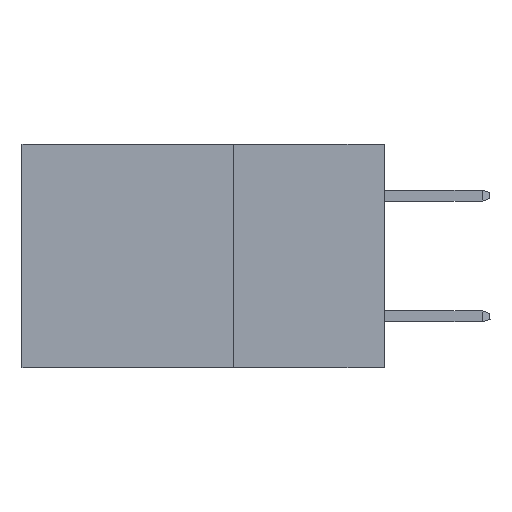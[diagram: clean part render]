
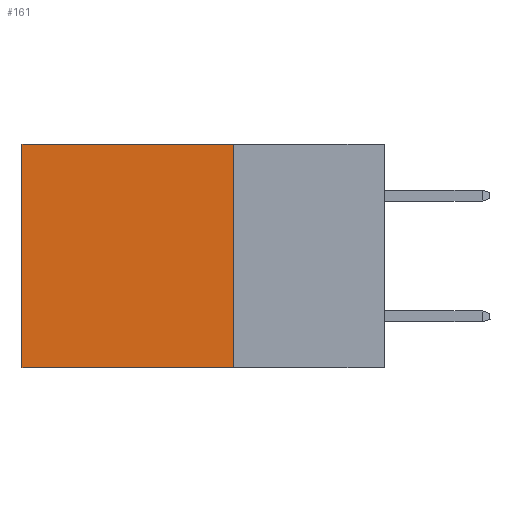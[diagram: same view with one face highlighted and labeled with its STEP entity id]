
A CAD part, left-side view. The second image highlights one B-rep face of the part: STEP entity #161.
In plain terms, the highlighted planar face has unit normal (-1, 0, 0).
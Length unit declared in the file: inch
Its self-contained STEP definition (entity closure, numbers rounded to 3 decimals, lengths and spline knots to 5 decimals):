
#161 = ADVANCED_FACE ( 'NONE', ( #3444 ), #9119, .F. ) ;
#740 = VERTEX_POINT ( 'NONE', #3530 ) ;
#1201 = VERTEX_POINT ( 'NONE', #7461 ) ;
#1665 = AXIS2_PLACEMENT_3D ( 'NONE', #10880, #9931, #5651 ) ;
#2228 = CARTESIAN_POINT ( 'NONE',  ( 0.2615, 0.6, -0.37 ) ) ;
#2464 = CARTESIAN_POINT ( 'NONE',  ( 0.2615, 0.25, -0.37 ) ) ;
#3444 = FACE_OUTER_BOUND ( 'NONE', #10472, .T. ) ;
#3530 = CARTESIAN_POINT ( 'NONE',  ( 0.2615, 0.6, 0. ) ) ;
#3645 = LINE ( 'NONE', #2464, #8260 ) ;
#3822 = VECTOR ( 'NONE', #5399, 39.37008 ) ;
#4147 = ORIENTED_EDGE ( 'NONE', *, *, #4760, .T. ) ;
#4585 = CARTESIAN_POINT ( 'NONE',  ( 0.2615, 0.25, 0. ) ) ;
#4722 = VERTEX_POINT ( 'NONE', #4585 ) ;
#4760 = EDGE_CURVE ( 'NONE', #4722, #740, #6684, .T. ) ;
#5399 = DIRECTION ( 'NONE',  ( 0., 1., 0. ) ) ;
#5562 = EDGE_CURVE ( 'NONE', #8743, #1201, #8564, .T. ) ;
#5651 = DIRECTION ( 'NONE',  ( 0., 0., -1. ) ) ;
#6229 = ORIENTED_EDGE ( 'NONE', *, *, #6980, .T. ) ;
#6668 = CARTESIAN_POINT ( 'NONE',  ( 0.2615, 0.25, -0.37 ) ) ;
#6683 = DIRECTION ( 'NONE',  ( 0., 0., -1. ) ) ;
#6684 = LINE ( 'NONE', #7137, #3822 ) ;
#6980 = EDGE_CURVE ( 'NONE', #740, #1201, #11084, .T. ) ;
#7137 = CARTESIAN_POINT ( 'NONE',  ( 0.2615, 0.25, 0. ) ) ;
#7321 = CARTESIAN_POINT ( 'NONE',  ( 0.2615, 0.25, -0.37 ) ) ;
#7461 = CARTESIAN_POINT ( 'NONE',  ( 0.2615, 0.6, -0.37 ) ) ;
#8260 = VECTOR ( 'NONE', #8625, 39.37008 ) ;
#8398 = DIRECTION ( 'NONE',  ( 0., 1., 0. ) ) ;
#8564 = LINE ( 'NONE', #6668, #10363 ) ;
#8625 = DIRECTION ( 'NONE',  ( 0., 0., -1. ) ) ;
#8743 = VERTEX_POINT ( 'NONE', #7321 ) ;
#8790 = ORIENTED_EDGE ( 'NONE', *, *, #10725, .F. ) ;
#9119 = PLANE ( 'NONE',  #1665 ) ;
#9484 = ORIENTED_EDGE ( 'NONE', *, *, #5562, .F. ) ;
#9931 = DIRECTION ( 'NONE',  ( 1., 0., 0. ) ) ;
#10363 = VECTOR ( 'NONE', #8398, 39.37008 ) ;
#10472 = EDGE_LOOP ( 'NONE', ( #6229, #9484, #8790, #4147 ) ) ;
#10725 = EDGE_CURVE ( 'NONE', #4722, #8743, #3645, .T. ) ;
#10880 = CARTESIAN_POINT ( 'NONE',  ( 0.2615, 0.25, -0.37 ) ) ;
#11084 = LINE ( 'NONE', #2228, #11227 ) ;
#11227 = VECTOR ( 'NONE', #6683, 39.37008 ) ;
